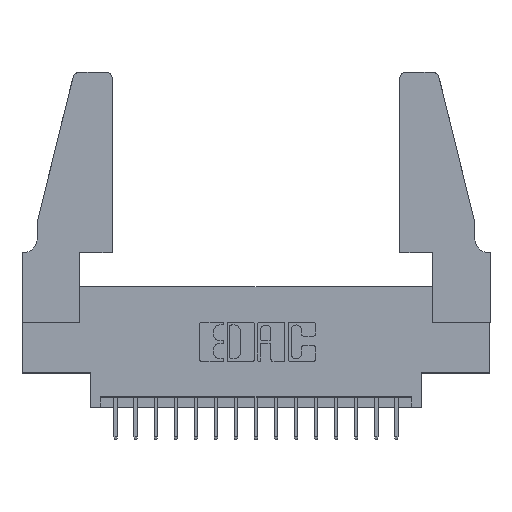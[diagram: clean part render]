
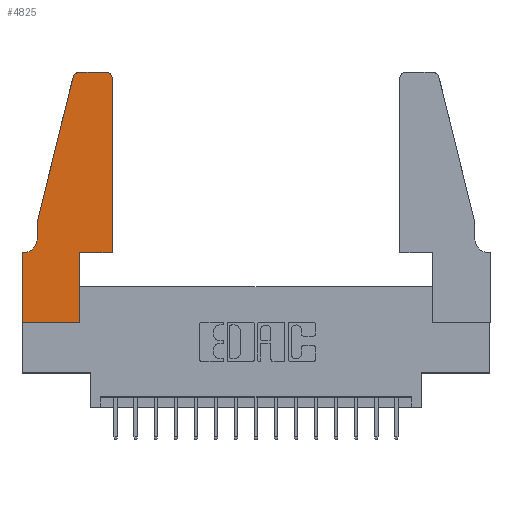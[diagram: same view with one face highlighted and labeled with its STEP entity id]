
A CAD part, top view. The second image highlights one B-rep face of the part: STEP entity #4825.
In plain terms, the highlighted planar face has unit normal (0, 0, 1).
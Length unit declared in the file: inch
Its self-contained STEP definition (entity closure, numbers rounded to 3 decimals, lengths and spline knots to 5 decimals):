
#49 = CARTESIAN_POINT ( 'NONE',  ( 0.2865, 0.35, 0.37 ) ) ;
#236 = VECTOR ( 'NONE', #3432, 39.37008 ) ;
#254 = DIRECTION ( 'NONE',  ( -1., 0., 0. ) ) ;
#266 = CARTESIAN_POINT ( 'NONE',  ( 0., 0.35, 0.37 ) ) ;
#326 = CARTESIAN_POINT ( 'NONE',  ( 0.4205, 1.25, 0.37 ) ) ;
#355 = ORIENTED_EDGE ( 'NONE', *, *, #2986, .T. ) ;
#730 = EDGE_CURVE ( 'NONE', #8214, #4809, #5657, .T. ) ;
#1370 = DIRECTION ( 'NONE',  ( 0., 1., 0. ) ) ;
#1408 = CIRCLE ( 'NONE', #7269, 0.03 ) ;
#1712 = DIRECTION ( 'NONE',  ( 1., 0., 0. ) ) ;
#1880 = CARTESIAN_POINT ( 'NONE',  ( 0.4505, 0.35, 0.37 ) ) ;
#1996 = ORIENTED_EDGE ( 'NONE', *, *, #8113, .T. ) ;
#1997 = CARTESIAN_POINT ( 'NONE',  ( 0., 0.35, 0.37 ) ) ;
#2087 = EDGE_CURVE ( 'NONE', #9471, #9285, #16775, .T. ) ;
#2129 = EDGE_CURVE ( 'NONE', #9285, #8214, #9702, .T. ) ;
#2185 = VERTEX_POINT ( 'NONE', #1997 ) ;
#2196 = VECTOR ( 'NONE', #15444, 39.37008 ) ;
#2755 = CARTESIAN_POINT ( 'NONE',  ( 0., 0., 0.37 ) ) ;
#2940 = DIRECTION ( 'NONE',  ( 0., 0., 1. ) ) ;
#2986 = EDGE_CURVE ( 'NONE', #4809, #17584, #17575, .T. ) ;
#3090 = ORIENTED_EDGE ( 'NONE', *, *, #9325, .T. ) ;
#3110 = CARTESIAN_POINT ( 'NONE',  ( 0.0755, 0.35, 0.37 ) ) ;
#3432 = DIRECTION ( 'NONE',  ( 1., 0., 0. ) ) ;
#3518 = DIRECTION ( 'NONE',  ( -1., 0., 0. ) ) ;
#3605 = VERTEX_POINT ( 'NONE', #2755 ) ;
#4127 = VECTOR ( 'NONE', #6496, 39.37008 ) ;
#4563 = CARTESIAN_POINT ( 'NONE',  ( 0.2865, 0.35, 0.37 ) ) ;
#4783 = CARTESIAN_POINT ( 'NONE',  ( 0.0055, 0.42, 0.37 ) ) ;
#4809 = VERTEX_POINT ( 'NONE', #14119 ) ;
#4813 = CARTESIAN_POINT ( 'NONE',  ( 0.25487, 1.22718, 0.37 ) ) ;
#4825 = ADVANCED_FACE ( 'NONE', ( #15912 ), #7398, .T. ) ;
#4927 = VERTEX_POINT ( 'NONE', #16987 ) ;
#4977 = VECTOR ( 'NONE', #1370, 39.37008 ) ;
#5063 = ORIENTED_EDGE ( 'NONE', *, *, #6715, .T. ) ;
#5157 = DIRECTION ( 'NONE',  ( 0., -1., 0. ) ) ;
#5223 = CARTESIAN_POINT ( 'NONE',  ( 0.4505, 0.35, 0.37 ) ) ;
#5422 = LINE ( 'NONE', #11184, #4977 ) ;
#5657 = LINE ( 'NONE', #9375, #16019 ) ;
#6008 = LINE ( 'NONE', #4563, #2196 ) ;
#6045 = VECTOR ( 'NONE', #3518, 39.37008 ) ;
#6072 = VERTEX_POINT ( 'NONE', #49 ) ;
#6197 = DIRECTION ( 'NONE',  ( -1., 0., 0. ) ) ;
#6225 = EDGE_CURVE ( 'NONE', #17584, #16983, #16125, .T. ) ;
#6496 = DIRECTION ( 'NONE',  ( 0., -1., 0. ) ) ;
#6525 = VECTOR ( 'NONE', #11675, 39.37008 ) ;
#6578 = LINE ( 'NONE', #13247, #4127 ) ;
#6715 = EDGE_CURVE ( 'NONE', #4927, #6072, #6008, .T. ) ;
#6861 = ORIENTED_EDGE ( 'NONE', *, *, #730, .T. ) ;
#6902 = CARTESIAN_POINT ( 'NONE',  ( 0.4505, 1.22, 0.37 ) ) ;
#7269 = AXIS2_PLACEMENT_3D ( 'NONE', #11285, #2940, #12624 ) ;
#7398 = PLANE ( 'NONE',  #9623 ) ;
#7460 = DIRECTION ( 'NONE',  ( -0.239, -0.971, 0. ) ) ;
#7563 = CARTESIAN_POINT ( 'NONE',  ( 0.284, 1.22, 0.37 ) ) ;
#7846 = ORIENTED_EDGE ( 'NONE', *, *, #9674, .T. ) ;
#7895 = DIRECTION ( 'NONE',  ( 1., 0., 0. ) ) ;
#8113 = EDGE_CURVE ( 'NONE', #16983, #2185, #16697, .T. ) ;
#8214 = VERTEX_POINT ( 'NONE', #4813 ) ;
#8276 = LINE ( 'NONE', #8985, #236 ) ;
#8934 = ORIENTED_EDGE ( 'NONE', *, *, #11026, .T. ) ;
#8985 = CARTESIAN_POINT ( 'NONE',  ( 0., 0., 0.37 ) ) ;
#9285 = VERTEX_POINT ( 'NONE', #13121 ) ;
#9325 = EDGE_CURVE ( 'NONE', #16097, #9471, #1408, .T. ) ;
#9375 = CARTESIAN_POINT ( 'NONE',  ( 0.0755, 0.5, 0.37 ) ) ;
#9471 = VERTEX_POINT ( 'NONE', #326 ) ;
#9623 = AXIS2_PLACEMENT_3D ( 'NONE', #266, #10130, #1712 ) ;
#9674 = EDGE_CURVE ( 'NONE', #2185, #3605, #6578, .T. ) ;
#9702 = CIRCLE ( 'NONE', #11429, 0.03 ) ;
#10085 = CARTESIAN_POINT ( 'NONE',  ( 0.2605, 1.25, 0.37 ) ) ;
#10130 = DIRECTION ( 'NONE',  ( 0., 0., 1. ) ) ;
#10491 = ORIENTED_EDGE ( 'NONE', *, *, #2087, .T. ) ;
#10547 = EDGE_LOOP ( 'NONE', ( #10491, #16606, #6861, #355, #15009, #1996, #7846, #15385, #5063, #8934, #17099, #3090 ) ) ;
#11026 = EDGE_CURVE ( 'NONE', #6072, #11275, #17625, .T. ) ;
#11184 = CARTESIAN_POINT ( 'NONE',  ( 0.4505, 0.35, 0.37 ) ) ;
#11275 = VERTEX_POINT ( 'NONE', #5223 ) ;
#11285 = CARTESIAN_POINT ( 'NONE',  ( 0.4205, 1.22, 0.37 ) ) ;
#11429 = AXIS2_PLACEMENT_3D ( 'NONE', #7563, #16791, #7895 ) ;
#11541 = CARTESIAN_POINT ( 'NONE',  ( 0.0055, 0.35, 0.37 ) ) ;
#11675 = DIRECTION ( 'NONE',  ( 1., 0., 0. ) ) ;
#12624 = DIRECTION ( 'NONE',  ( 1., 0., 0. ) ) ;
#12729 = CARTESIAN_POINT ( 'NONE',  ( 0.0755, 0.42, 0.37 ) ) ;
#13121 = CARTESIAN_POINT ( 'NONE',  ( 0.284, 1.25, 0.37 ) ) ;
#13196 = VECTOR ( 'NONE', #254, 39.37008 ) ;
#13247 = CARTESIAN_POINT ( 'NONE',  ( 0., 0., 0.37 ) ) ;
#13684 = AXIS2_PLACEMENT_3D ( 'NONE', #4783, #14300, #6197 ) ;
#13838 = EDGE_CURVE ( 'NONE', #3605, #4927, #8276, .T. ) ;
#14119 = CARTESIAN_POINT ( 'NONE',  ( 0.0755, 0.5, 0.37 ) ) ;
#14240 = EDGE_CURVE ( 'NONE', #11275, #16097, #5422, .T. ) ;
#14300 = DIRECTION ( 'NONE',  ( 0., 0., -1. ) ) ;
#14492 = VECTOR ( 'NONE', #5157, 39.37008 ) ;
#14604 = CARTESIAN_POINT ( 'NONE',  ( 0.0755, 0.5, 0.37 ) ) ;
#15009 = ORIENTED_EDGE ( 'NONE', *, *, #6225, .T. ) ;
#15385 = ORIENTED_EDGE ( 'NONE', *, *, #13838, .T. ) ;
#15444 = DIRECTION ( 'NONE',  ( 0., 1., 0. ) ) ;
#15912 = FACE_OUTER_BOUND ( 'NONE', #10547, .T. ) ;
#16019 = VECTOR ( 'NONE', #7460, 39.37008 ) ;
#16097 = VERTEX_POINT ( 'NONE', #6902 ) ;
#16125 = CIRCLE ( 'NONE', #13684, 0.07 ) ;
#16606 = ORIENTED_EDGE ( 'NONE', *, *, #2129, .T. ) ;
#16697 = LINE ( 'NONE', #3110, #13196 ) ;
#16775 = LINE ( 'NONE', #10085, #6045 ) ;
#16791 = DIRECTION ( 'NONE',  ( 0., 0., 1. ) ) ;
#16983 = VERTEX_POINT ( 'NONE', #11541 ) ;
#16987 = CARTESIAN_POINT ( 'NONE',  ( 0.2865, 0., 0.37 ) ) ;
#17099 = ORIENTED_EDGE ( 'NONE', *, *, #14240, .T. ) ;
#17575 = LINE ( 'NONE', #14604, #14492 ) ;
#17584 = VERTEX_POINT ( 'NONE', #12729 ) ;
#17625 = LINE ( 'NONE', #1880, #6525 ) ;
